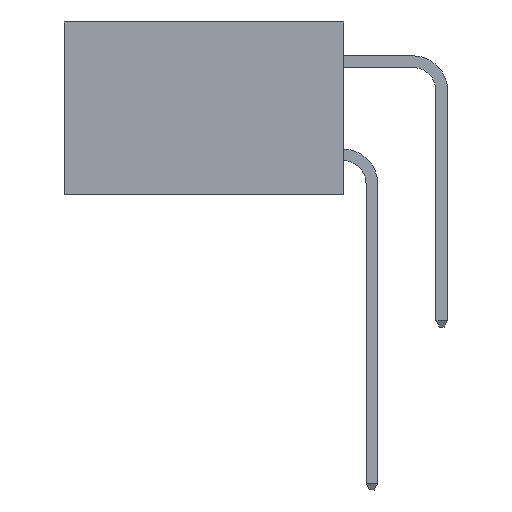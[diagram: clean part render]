
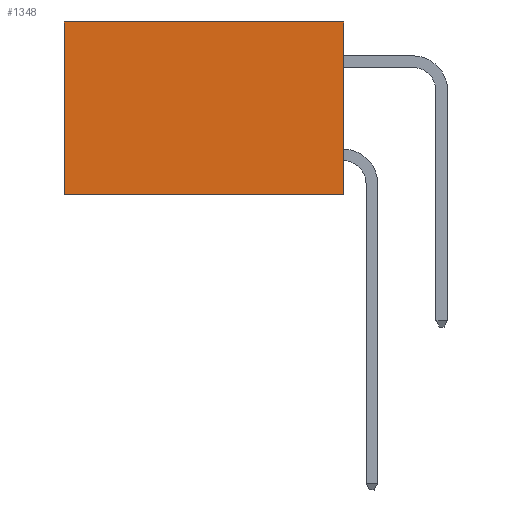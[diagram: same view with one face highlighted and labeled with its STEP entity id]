
A CAD part, left-side view. The second image highlights one B-rep face of the part: STEP entity #1348.
In plain terms, the highlighted planar face has unit normal (-1, 0, 0).
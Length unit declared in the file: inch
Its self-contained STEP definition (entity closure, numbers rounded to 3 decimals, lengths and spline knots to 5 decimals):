
#950 = AXIS2_PLACEMENT_3D ( 'NONE', #3628, #6723, #10303 ) ;
#1231 = EDGE_CURVE ( 'NONE', #14131, #16870, #12938, .T. ) ;
#1348 = ADVANCED_FACE ( 'NONE', ( #3534 ), #19776, .F. ) ;
#1406 = CARTESIAN_POINT ( 'NONE',  ( 0.2615, 0.6, 0. ) ) ;
#1466 = VECTOR ( 'NONE', #2504, 39.37008 ) ;
#1778 = VECTOR ( 'NONE', #3817, 39.37008 ) ;
#2504 = DIRECTION ( 'NONE',  ( 0., 1., 0. ) ) ;
#3534 = FACE_OUTER_BOUND ( 'NONE', #12127, .T. ) ;
#3628 = CARTESIAN_POINT ( 'NONE',  ( 0.2615, 0., -0.37 ) ) ;
#3817 = DIRECTION ( 'NONE',  ( 0., 0., -1. ) ) ;
#3990 = CARTESIAN_POINT ( 'NONE',  ( 0.2615, 0., 0. ) ) ;
#4052 = EDGE_CURVE ( 'NONE', #13560, #16870, #12318, .T. ) ;
#4707 = CARTESIAN_POINT ( 'NONE',  ( 0.2615, 0.6, -0.37 ) ) ;
#6723 = DIRECTION ( 'NONE',  ( 1., 0., 0. ) ) ;
#7280 = LINE ( 'NONE', #3990, #1466 ) ;
#8474 = ORIENTED_EDGE ( 'NONE', *, *, #17731, .F. ) ;
#9635 = EDGE_CURVE ( 'NONE', #11920, #14131, #7280, .T. ) ;
#10161 = LINE ( 'NONE', #16579, #1778 ) ;
#10303 = DIRECTION ( 'NONE',  ( 0., 0., -1. ) ) ;
#10734 = DIRECTION ( 'NONE',  ( 0., 1., 0. ) ) ;
#11074 = VECTOR ( 'NONE', #14204, 39.37008 ) ;
#11920 = VERTEX_POINT ( 'NONE', #19801 ) ;
#12127 = EDGE_LOOP ( 'NONE', ( #17374, #16140, #8474, #18667 ) ) ;
#12318 = LINE ( 'NONE', #18723, #20076 ) ;
#12825 = CARTESIAN_POINT ( 'NONE',  ( 0.2615, 0.6, -0.37 ) ) ;
#12938 = LINE ( 'NONE', #4707, #11074 ) ;
#13560 = VERTEX_POINT ( 'NONE', #15508 ) ;
#14131 = VERTEX_POINT ( 'NONE', #1406 ) ;
#14204 = DIRECTION ( 'NONE',  ( 0., 0., -1. ) ) ;
#15508 = CARTESIAN_POINT ( 'NONE',  ( 0.2615, 0., -0.37 ) ) ;
#16140 = ORIENTED_EDGE ( 'NONE', *, *, #4052, .F. ) ;
#16579 = CARTESIAN_POINT ( 'NONE',  ( 0.2615, 0., -0.37 ) ) ;
#16870 = VERTEX_POINT ( 'NONE', #12825 ) ;
#17374 = ORIENTED_EDGE ( 'NONE', *, *, #1231, .T. ) ;
#17731 = EDGE_CURVE ( 'NONE', #11920, #13560, #10161, .T. ) ;
#18667 = ORIENTED_EDGE ( 'NONE', *, *, #9635, .T. ) ;
#18723 = CARTESIAN_POINT ( 'NONE',  ( 0.2615, 0., -0.37 ) ) ;
#19776 = PLANE ( 'NONE',  #950 ) ;
#19801 = CARTESIAN_POINT ( 'NONE',  ( 0.2615, 0., 0. ) ) ;
#20076 = VECTOR ( 'NONE', #10734, 39.37008 ) ;
